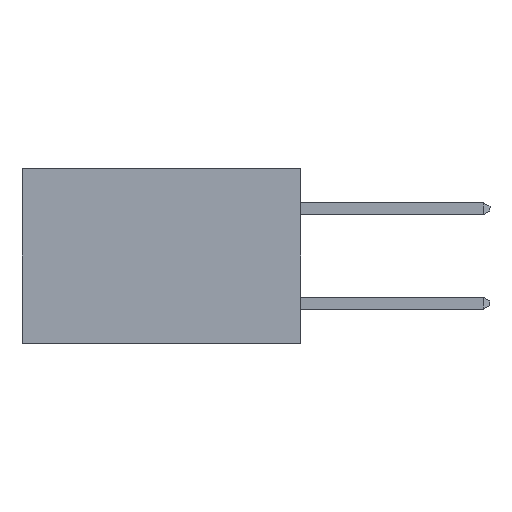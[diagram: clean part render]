
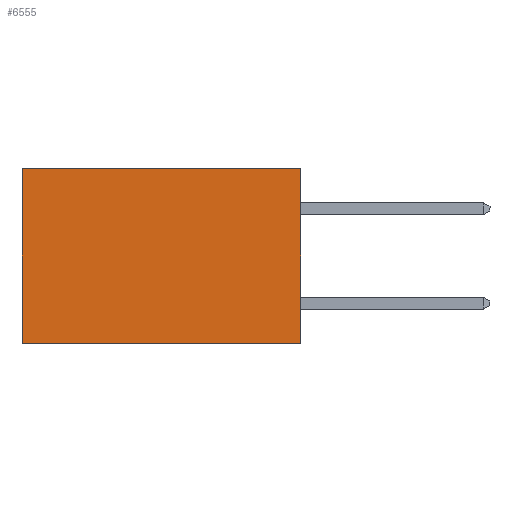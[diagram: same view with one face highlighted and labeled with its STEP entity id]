
A CAD part, left-side view. The second image highlights one B-rep face of the part: STEP entity #6555.
In plain terms, the highlighted planar face has unit normal (-1, 0, 0).
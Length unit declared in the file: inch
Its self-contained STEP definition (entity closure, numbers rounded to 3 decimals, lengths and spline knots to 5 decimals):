
#48 = VERTEX_POINT ( 'NONE', #8869 ) ;
#404 = VERTEX_POINT ( 'NONE', #11529 ) ;
#495 = DIRECTION ( 'NONE',  ( 0., 0., -1. ) ) ;
#603 = LINE ( 'NONE', #5325, #8702 ) ;
#722 = CARTESIAN_POINT ( 'NONE',  ( 0.277, 0., -0.37 ) ) ;
#1124 = DIRECTION ( 'NONE',  ( 0., 0., -1. ) ) ;
#1137 = DIRECTION ( 'NONE',  ( 1., 0., 0. ) ) ;
#1307 = CARTESIAN_POINT ( 'NONE',  ( 0.277, 0., -0.37 ) ) ;
#1348 = VERTEX_POINT ( 'NONE', #8014 ) ;
#1371 = PLANE ( 'NONE',  #4962 ) ;
#2661 = EDGE_CURVE ( 'NONE', #7468, #48, #9915, .T. ) ;
#2692 = EDGE_CURVE ( 'NONE', #404, #48, #7690, .T. ) ;
#3270 = EDGE_LOOP ( 'NONE', ( #10120, #9552, #7733, #6594 ) ) ;
#3989 = VECTOR ( 'NONE', #9862, 39.37008 ) ;
#4314 = VECTOR ( 'NONE', #8164, 39.37008 ) ;
#4962 = AXIS2_PLACEMENT_3D ( 'NONE', #1307, #1137, #1124 ) ;
#5325 = CARTESIAN_POINT ( 'NONE',  ( 0.277, 0., 0. ) ) ;
#5753 = EDGE_CURVE ( 'NONE', #1348, #7468, #7272, .T. ) ;
#6403 = CARTESIAN_POINT ( 'NONE',  ( 0.277, 0., -0.37 ) ) ;
#6555 = ADVANCED_FACE ( 'NONE', ( #11396 ), #1371, .F. ) ;
#6594 = ORIENTED_EDGE ( 'NONE', *, *, #11899, .T. ) ;
#7272 = LINE ( 'NONE', #722, #12709 ) ;
#7468 = VERTEX_POINT ( 'NONE', #6403 ) ;
#7690 = LINE ( 'NONE', #9875, #3989 ) ;
#7733 = ORIENTED_EDGE ( 'NONE', *, *, #5753, .F. ) ;
#8014 = CARTESIAN_POINT ( 'NONE',  ( 0.277, 0., 0. ) ) ;
#8164 = DIRECTION ( 'NONE',  ( 0., 1., 0. ) ) ;
#8702 = VECTOR ( 'NONE', #9513, 39.37008 ) ;
#8849 = CARTESIAN_POINT ( 'NONE',  ( 0.277, 0., -0.37 ) ) ;
#8869 = CARTESIAN_POINT ( 'NONE',  ( 0.277, 0.59, -0.37 ) ) ;
#9513 = DIRECTION ( 'NONE',  ( 0., 1., 0. ) ) ;
#9552 = ORIENTED_EDGE ( 'NONE', *, *, #2661, .F. ) ;
#9862 = DIRECTION ( 'NONE',  ( 0., 0., -1. ) ) ;
#9875 = CARTESIAN_POINT ( 'NONE',  ( 0.277, 0.59, -0.37 ) ) ;
#9915 = LINE ( 'NONE', #8849, #4314 ) ;
#10120 = ORIENTED_EDGE ( 'NONE', *, *, #2692, .T. ) ;
#11396 = FACE_OUTER_BOUND ( 'NONE', #3270, .T. ) ;
#11529 = CARTESIAN_POINT ( 'NONE',  ( 0.277, 0.59, 0. ) ) ;
#11899 = EDGE_CURVE ( 'NONE', #1348, #404, #603, .T. ) ;
#12709 = VECTOR ( 'NONE', #495, 39.37008 ) ;
